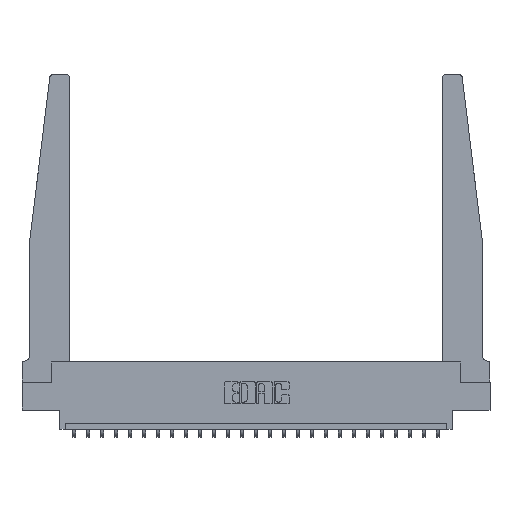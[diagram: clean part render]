
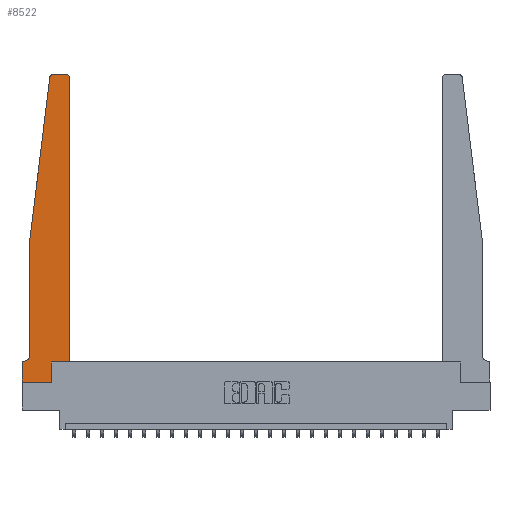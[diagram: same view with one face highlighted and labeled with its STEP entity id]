
A CAD part, top view. The second image highlights one B-rep face of the part: STEP entity #8522.
In plain terms, the highlighted planar face has unit normal (0, 0, 1).
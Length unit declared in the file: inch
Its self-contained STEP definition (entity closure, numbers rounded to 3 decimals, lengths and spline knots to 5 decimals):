
#328 = DIRECTION ( 'NONE',  ( 0., 1., 0. ) ) ;
#734 = EDGE_CURVE ( 'NONE', #2755, #18698, #19914, .T. ) ;
#879 = LINE ( 'NONE', #3957, #19835 ) ;
#889 = AXIS2_PLACEMENT_3D ( 'NONE', #19793, #8821, #21629 ) ;
#1131 = VECTOR ( 'NONE', #5894, 39.37008 ) ;
#1214 = CARTESIAN_POINT ( 'NONE',  ( 0., 0.1875, 0.37 ) ) ;
#1615 = DIRECTION ( 'NONE',  ( 1., 0., 0. ) ) ;
#1654 = CARTESIAN_POINT ( 'NONE',  ( 0.065, 1.25, 0.37 ) ) ;
#1713 = ORIENTED_EDGE ( 'NONE', *, *, #734, .T. ) ;
#2049 = CIRCLE ( 'NONE', #19193, 0.03 ) ;
#2177 = ORIENTED_EDGE ( 'NONE', *, *, #9055, .T. ) ;
#2649 = FACE_OUTER_BOUND ( 'NONE', #10551, .T. ) ;
#2755 = VERTEX_POINT ( 'NONE', #10686 ) ;
#2893 = CARTESIAN_POINT ( 'NONE',  ( 0.015, 0.1875, 0.37 ) ) ;
#2905 = LINE ( 'NONE', #19102, #21818 ) ;
#3290 = ORIENTED_EDGE ( 'NONE', *, *, #9364, .T. ) ;
#3957 = CARTESIAN_POINT ( 'NONE',  ( 0.25, 2.75, 0.37 ) ) ;
#3960 = CARTESIAN_POINT ( 'NONE',  ( 0.425, 0.18, 0.37 ) ) ;
#4254 = VECTOR ( 'NONE', #16445, 39.37008 ) ;
#5396 = EDGE_CURVE ( 'NONE', #21675, #16249, #13940, .T. ) ;
#5504 = VECTOR ( 'NONE', #20848, 39.37008 ) ;
#5567 = EDGE_CURVE ( 'NONE', #15925, #8563, #11056, .T. ) ;
#5611 = DIRECTION ( 'NONE',  ( 0., 0., 1. ) ) ;
#5894 = DIRECTION ( 'NONE',  ( -1., 0., 0. ) ) ;
#6250 = VECTOR ( 'NONE', #15886, 39.37008 ) ;
#6309 = ORIENTED_EDGE ( 'NONE', *, *, #21202, .T. ) ;
#6657 = ORIENTED_EDGE ( 'NONE', *, *, #13510, .T. ) ;
#7387 = AXIS2_PLACEMENT_3D ( 'NONE', #16531, #5611, #18377 ) ;
#7852 = EDGE_CURVE ( 'NONE', #15121, #16388, #17564, .T. ) ;
#8175 = CARTESIAN_POINT ( 'NONE',  ( 0.395, 2.72, 0.37 ) ) ;
#8522 = ADVANCED_FACE ( 'NONE', ( #2649 ), #12854, .T. ) ;
#8563 = VERTEX_POINT ( 'NONE', #16619 ) ;
#8673 = CARTESIAN_POINT ( 'NONE',  ( 0.065, 1.25, 0.37 ) ) ;
#8821 = DIRECTION ( 'NONE',  ( 0., 0., -1. ) ) ;
#8840 = ORIENTED_EDGE ( 'NONE', *, *, #18242, .T. ) ;
#9055 = EDGE_CURVE ( 'NONE', #13684, #13418, #2049, .T. ) ;
#9182 = ORIENTED_EDGE ( 'NONE', *, *, #12123, .T. ) ;
#9364 = EDGE_CURVE ( 'NONE', #8563, #2755, #9781, .T. ) ;
#9395 = LINE ( 'NONE', #1654, #13690 ) ;
#9415 = DIRECTION ( 'NONE',  ( 1., 0., 0. ) ) ;
#9500 = CARTESIAN_POINT ( 'NONE',  ( 0.425, 0.18, 0.37 ) ) ;
#9781 = LINE ( 'NONE', #15314, #5504 ) ;
#9833 = EDGE_CURVE ( 'NONE', #16388, #15861, #10894, .T. ) ;
#9941 = CARTESIAN_POINT ( 'NONE',  ( 0.395, 2.75, 0.37 ) ) ;
#9993 = DIRECTION ( 'NONE',  ( 1., 0., 0. ) ) ;
#10118 = CARTESIAN_POINT ( 'NONE',  ( 0.27653, 2.75, 0.37 ) ) ;
#10551 = EDGE_LOOP ( 'NONE', ( #9182, #2177, #6309, #8840, #21720, #16202, #16855, #17960, #3290, #1713, #6657, #10742 ) ) ;
#10686 = CARTESIAN_POINT ( 'NONE',  ( 0.2605, 0.18, 0.37 ) ) ;
#10742 = ORIENTED_EDGE ( 'NONE', *, *, #5396, .T. ) ;
#10894 = LINE ( 'NONE', #18645, #1131 ) ;
#11056 = LINE ( 'NONE', #14067, #6250 ) ;
#11158 = VECTOR ( 'NONE', #328, 39.37008 ) ;
#12123 = EDGE_CURVE ( 'NONE', #16249, #13684, #879, .T. ) ;
#12596 = DIRECTION ( 'NONE',  ( 0., 0., 1. ) ) ;
#12854 = PLANE ( 'NONE',  #7387 ) ;
#13418 = VERTEX_POINT ( 'NONE', #22064 ) ;
#13510 = EDGE_CURVE ( 'NONE', #18698, #21675, #20906, .T. ) ;
#13684 = VERTEX_POINT ( 'NONE', #10118 ) ;
#13690 = VECTOR ( 'NONE', #16307, 39.37008 ) ;
#13940 = CIRCLE ( 'NONE', #18051, 0.03 ) ;
#14067 = CARTESIAN_POINT ( 'NONE',  ( 0., 0., 0.37 ) ) ;
#14196 = CARTESIAN_POINT ( 'NONE',  ( 0., 0., 0.37 ) ) ;
#14624 = CARTESIAN_POINT ( 'NONE',  ( 0., 0., 0.37 ) ) ;
#15049 = VECTOR ( 'NONE', #9415, 39.37008 ) ;
#15121 = VERTEX_POINT ( 'NONE', #17972 ) ;
#15314 = CARTESIAN_POINT ( 'NONE',  ( 0.2605, 0.18, 0.37 ) ) ;
#15500 = EDGE_CURVE ( 'NONE', #15861, #15925, #18839, .T. ) ;
#15861 = VERTEX_POINT ( 'NONE', #1214 ) ;
#15886 = DIRECTION ( 'NONE',  ( 1., 0., 0. ) ) ;
#15925 = VERTEX_POINT ( 'NONE', #14196 ) ;
#16202 = ORIENTED_EDGE ( 'NONE', *, *, #9833, .T. ) ;
#16249 = VERTEX_POINT ( 'NONE', #9941 ) ;
#16307 = DIRECTION ( 'NONE',  ( -0.122, -0.992, 0. ) ) ;
#16388 = VERTEX_POINT ( 'NONE', #2893 ) ;
#16445 = DIRECTION ( 'NONE',  ( 0., -1., 0. ) ) ;
#16531 = CARTESIAN_POINT ( 'NONE',  ( 0., 0.1875, 0.37 ) ) ;
#16619 = CARTESIAN_POINT ( 'NONE',  ( 0.2605, 0., 0.37 ) ) ;
#16855 = ORIENTED_EDGE ( 'NONE', *, *, #15500, .T. ) ;
#17564 = CIRCLE ( 'NONE', #889, 0.05 ) ;
#17651 = CARTESIAN_POINT ( 'NONE',  ( 0.425, 2.72, 0.37 ) ) ;
#17960 = ORIENTED_EDGE ( 'NONE', *, *, #5567, .T. ) ;
#17972 = CARTESIAN_POINT ( 'NONE',  ( 0.065, 0.2375, 0.37 ) ) ;
#18051 = AXIS2_PLACEMENT_3D ( 'NONE', #8175, #20980, #9993 ) ;
#18242 = EDGE_CURVE ( 'NONE', #23240, #15121, #2905, .T. ) ;
#18377 = DIRECTION ( 'NONE',  ( 1., 0., 0. ) ) ;
#18645 = CARTESIAN_POINT ( 'NONE',  ( 0.065, 0.1875, 0.37 ) ) ;
#18698 = VERTEX_POINT ( 'NONE', #3960 ) ;
#18839 = LINE ( 'NONE', #14624, #4254 ) ;
#19102 = CARTESIAN_POINT ( 'NONE',  ( 0.065, 1.25, 0.37 ) ) ;
#19193 = AXIS2_PLACEMENT_3D ( 'NONE', #23562, #12596, #1615 ) ;
#19793 = CARTESIAN_POINT ( 'NONE',  ( 0.015, 0.2375, 0.37 ) ) ;
#19835 = VECTOR ( 'NONE', #20444, 39.37008 ) ;
#19914 = LINE ( 'NONE', #23289, #15049 ) ;
#20444 = DIRECTION ( 'NONE',  ( -1., 0., 0. ) ) ;
#20848 = DIRECTION ( 'NONE',  ( 0., 1., 0. ) ) ;
#20906 = LINE ( 'NONE', #9500, #11158 ) ;
#20959 = DIRECTION ( 'NONE',  ( 0., -1., 0. ) ) ;
#20980 = DIRECTION ( 'NONE',  ( 0., 0., 1. ) ) ;
#21202 = EDGE_CURVE ( 'NONE', #13418, #23240, #9395, .T. ) ;
#21629 = DIRECTION ( 'NONE',  ( -1., 0., 0. ) ) ;
#21675 = VERTEX_POINT ( 'NONE', #17651 ) ;
#21720 = ORIENTED_EDGE ( 'NONE', *, *, #7852, .T. ) ;
#21818 = VECTOR ( 'NONE', #20959, 39.37008 ) ;
#22064 = CARTESIAN_POINT ( 'NONE',  ( 0.24675, 2.72367, 0.37 ) ) ;
#23240 = VERTEX_POINT ( 'NONE', #8673 ) ;
#23289 = CARTESIAN_POINT ( 'NONE',  ( 0.425, 0.18, 0.37 ) ) ;
#23562 = CARTESIAN_POINT ( 'NONE',  ( 0.27653, 2.72, 0.37 ) ) ;
